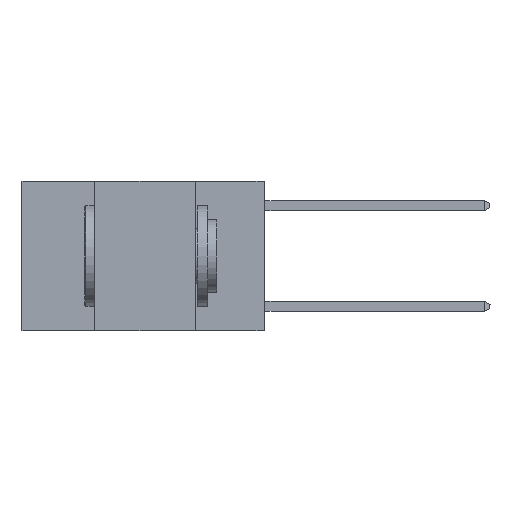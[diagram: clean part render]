
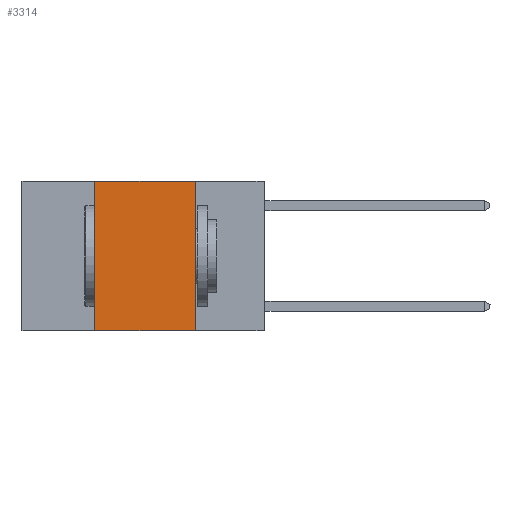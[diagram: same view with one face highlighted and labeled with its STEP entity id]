
A CAD part, left-side view. The second image highlights one B-rep face of the part: STEP entity #3314.
In plain terms, the highlighted planar face has unit normal (-1, 0, 0).
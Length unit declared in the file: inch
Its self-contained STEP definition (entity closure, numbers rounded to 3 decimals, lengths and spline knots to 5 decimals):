
#1708 = VERTEX_POINT ( 'NONE', #9070 ) ;
#2855 = CARTESIAN_POINT ( 'NONE',  ( 0., 0.42, 0. ) ) ;
#2975 = VERTEX_POINT ( 'NONE', #24888 ) ;
#3122 = ORIENTED_EDGE ( 'NONE', *, *, #6877, .F. ) ;
#3150 = DIRECTION ( 'NONE',  ( 0., -1., 0. ) ) ;
#3174 = PLANE ( 'NONE',  #28601 ) ;
#3176 = LINE ( 'NONE', #26386, #8699 ) ;
#3314 = ADVANCED_FACE ( 'NONE', ( #20866 ), #3174, .F. ) ;
#6877 = EDGE_CURVE ( 'NONE', #2975, #25266, #30146, .T. ) ;
#7606 = DIRECTION ( 'NONE',  ( 0., 0., 1. ) ) ;
#7912 = DIRECTION ( 'NONE',  ( 0., 0., -1. ) ) ;
#8699 = VECTOR ( 'NONE', #17145, 39.37008 ) ;
#9016 = VECTOR ( 'NONE', #3150, 39.37008 ) ;
#9070 = CARTESIAN_POINT ( 'NONE',  ( 0., 0.42, 0. ) ) ;
#12598 = CARTESIAN_POINT ( 'NONE',  ( 0., 0.42, -0.37 ) ) ;
#12661 = DIRECTION ( 'NONE',  ( 0., 0., -1. ) ) ;
#12682 = EDGE_LOOP ( 'NONE', ( #3122, #27050, #21975, #14741 ) ) ;
#14741 = ORIENTED_EDGE ( 'NONE', *, *, #29961, .T. ) ;
#15245 = LINE ( 'NONE', #28818, #9016 ) ;
#17145 = DIRECTION ( 'NONE',  ( 0., -1., 0. ) ) ;
#18503 = VECTOR ( 'NONE', #12661, 39.37008 ) ;
#19082 = EDGE_CURVE ( 'NONE', #29997, #1708, #28069, .T. ) ;
#19138 = EDGE_CURVE ( 'NONE', #1708, #2975, #3176, .T. ) ;
#19601 = CARTESIAN_POINT ( 'NONE',  ( 0., 0.6, 0. ) ) ;
#20866 = FACE_OUTER_BOUND ( 'NONE', #12682, .T. ) ;
#21888 = VECTOR ( 'NONE', #7606, 39.37008 ) ;
#21937 = DIRECTION ( 'NONE',  ( 1., 0., 0. ) ) ;
#21975 = ORIENTED_EDGE ( 'NONE', *, *, #19082, .F. ) ;
#22417 = CARTESIAN_POINT ( 'NONE',  ( 0., 0.17, -0.37 ) ) ;
#24888 = CARTESIAN_POINT ( 'NONE',  ( 0., 0.17, 0. ) ) ;
#25266 = VERTEX_POINT ( 'NONE', #22417 ) ;
#26386 = CARTESIAN_POINT ( 'NONE',  ( 0., 0.6, 0. ) ) ;
#27050 = ORIENTED_EDGE ( 'NONE', *, *, #19138, .F. ) ;
#28069 = LINE ( 'NONE', #2855, #21888 ) ;
#28601 = AXIS2_PLACEMENT_3D ( 'NONE', #19601, #21937, #7912 ) ;
#28818 = CARTESIAN_POINT ( 'NONE',  ( 0., 0.6, -0.37 ) ) ;
#28964 = CARTESIAN_POINT ( 'NONE',  ( 0., 0.17, 0. ) ) ;
#29961 = EDGE_CURVE ( 'NONE', #29997, #25266, #15245, .T. ) ;
#29997 = VERTEX_POINT ( 'NONE', #12598 ) ;
#30146 = LINE ( 'NONE', #28964, #18503 ) ;
